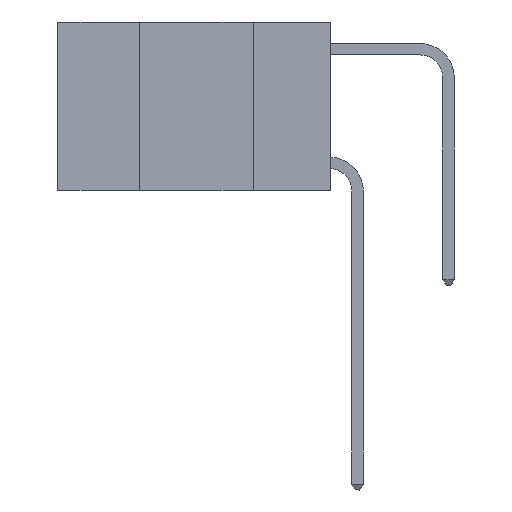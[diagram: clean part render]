
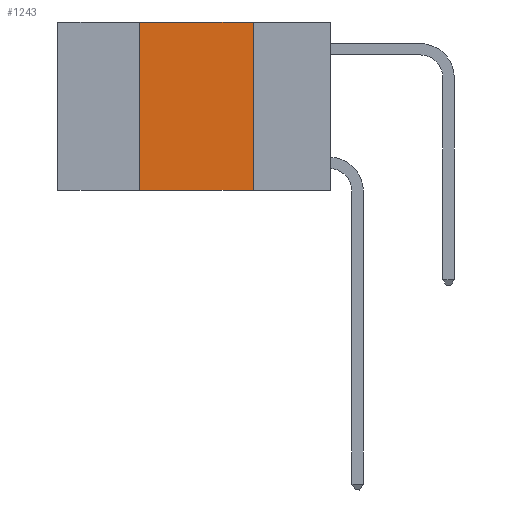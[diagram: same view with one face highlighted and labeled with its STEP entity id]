
A CAD part, left-side view. The second image highlights one B-rep face of the part: STEP entity #1243.
In plain terms, the highlighted planar face has unit normal (-1, 0, 0).
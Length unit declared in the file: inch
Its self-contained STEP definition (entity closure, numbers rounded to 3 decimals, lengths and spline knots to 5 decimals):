
#404 = CARTESIAN_POINT ( 'NONE',  ( 0., 0.17, -0.37 ) ) ;
#585 = VECTOR ( 'NONE', #12889, 39.37008 ) ;
#687 = AXIS2_PLACEMENT_3D ( 'NONE', #2663, #2685, #6628 ) ;
#731 = PLANE ( 'NONE',  #687 ) ;
#1191 = CARTESIAN_POINT ( 'NONE',  ( 0., 0.42, -0.37 ) ) ;
#1243 = ADVANCED_FACE ( 'NONE', ( #12386 ), #731, .F. ) ;
#1306 = DIRECTION ( 'NONE',  ( 0., 0., -1. ) ) ;
#1316 = VERTEX_POINT ( 'NONE', #404 ) ;
#1662 = DIRECTION ( 'NONE',  ( 0., -1., 0. ) ) ;
#2663 = CARTESIAN_POINT ( 'NONE',  ( 0., 0.6, 0. ) ) ;
#2685 = DIRECTION ( 'NONE',  ( 1., 0., 0. ) ) ;
#3792 = VERTEX_POINT ( 'NONE', #1191 ) ;
#3827 = VERTEX_POINT ( 'NONE', #12250 ) ;
#3848 = VECTOR ( 'NONE', #1306, 39.37008 ) ;
#4479 = CARTESIAN_POINT ( 'NONE',  ( 0., 0.17, 0. ) ) ;
#4717 = CARTESIAN_POINT ( 'NONE',  ( 0., 0.17, 0. ) ) ;
#6075 = CARTESIAN_POINT ( 'NONE',  ( 0., 0.42, 0. ) ) ;
#6537 = ORIENTED_EDGE ( 'NONE', *, *, #7269, .F. ) ;
#6628 = DIRECTION ( 'NONE',  ( 0., 0., -1. ) ) ;
#6666 = VECTOR ( 'NONE', #1662, 39.37008 ) ;
#7159 = EDGE_CURVE ( 'NONE', #10759, #1316, #9323, .T. ) ;
#7269 = EDGE_CURVE ( 'NONE', #3792, #3827, #11370, .T. ) ;
#7512 = EDGE_CURVE ( 'NONE', #3792, #1316, #9458, .T. ) ;
#7713 = LINE ( 'NONE', #9276, #12492 ) ;
#9276 = CARTESIAN_POINT ( 'NONE',  ( 0., 0.6, 0. ) ) ;
#9305 = ORIENTED_EDGE ( 'NONE', *, *, #10227, .F. ) ;
#9323 = LINE ( 'NONE', #4479, #3848 ) ;
#9458 = LINE ( 'NONE', #11672, #6666 ) ;
#10227 = EDGE_CURVE ( 'NONE', #3827, #10759, #7713, .T. ) ;
#10251 = DIRECTION ( 'NONE',  ( 0., -1., 0. ) ) ;
#10759 = VERTEX_POINT ( 'NONE', #4717 ) ;
#11214 = ORIENTED_EDGE ( 'NONE', *, *, #7159, .F. ) ;
#11370 = LINE ( 'NONE', #6075, #585 ) ;
#11672 = CARTESIAN_POINT ( 'NONE',  ( 0., 0.6, -0.37 ) ) ;
#11783 = EDGE_LOOP ( 'NONE', ( #11214, #9305, #6537, #11941 ) ) ;
#11941 = ORIENTED_EDGE ( 'NONE', *, *, #7512, .T. ) ;
#12250 = CARTESIAN_POINT ( 'NONE',  ( 0., 0.42, 0. ) ) ;
#12386 = FACE_OUTER_BOUND ( 'NONE', #11783, .T. ) ;
#12492 = VECTOR ( 'NONE', #10251, 39.37008 ) ;
#12889 = DIRECTION ( 'NONE',  ( 0., 0., 1. ) ) ;
